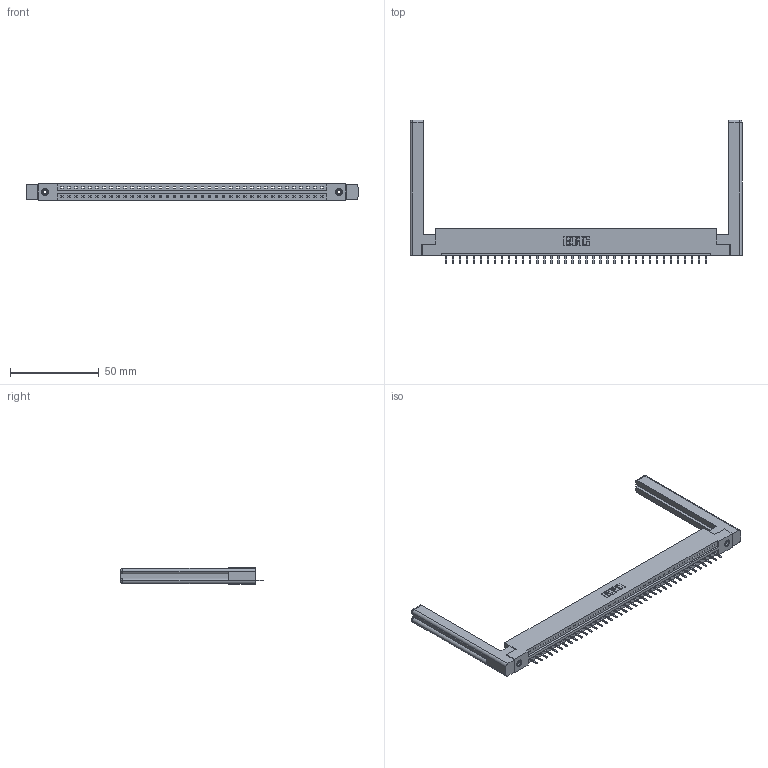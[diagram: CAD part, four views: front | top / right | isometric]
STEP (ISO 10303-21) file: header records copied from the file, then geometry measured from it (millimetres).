
FILE_DESCRIPTION (( 'STEP AP203' ), '1' );
FILE_NAME ('387-038-520-158.STEP', '2019-10-04T15:22:51', ( '' ), ( '' ), 'SwSTEP 2.0', 'SolidWorks 2016', '' );
FILE_SCHEMA (( 'CONFIG_CONTROL_DESIGN' ));
Length unit declared in the file: inch
Products named in the file (5): 307-220-058; 387-038-520-158; 337 Part_Flush Mounting Lugs - 0.156 Dia-TI; 345-292-001_345-293-120; 345-250-001_345-250-001-102
Assembly tree (43 placements, depth 2):
  387-038-520-158
    337 Part_Flush Mounting Lugs - 0.156 Dia-TI
    345-292-001_345-293-120  x38
    345-250-001_345-250-001-102  x2
    307-220-058  x2
Bounding box: 187.2 x 81.11 x 9.4 mm (x, y, z)
Volume: 26458.9 mm3; surface area: 24737.7 mm2
Topology: 43 solids, 43 shells, 2764 faces, 8113 edges, 5294 vertices
Faces by surface type: plane 1978, cylinder 762, cone 12, torus 12
Entity records: 31512 total; most frequent: CARTESIAN_POINT 5499, ORIENTED_EDGE 5400, DIRECTION 4644, EDGE_CURVE 2700, VECTOR 2520, LINE 2520, VERTEX_POINT 1790, AXIS2_PLACEMENT_3D 1062
